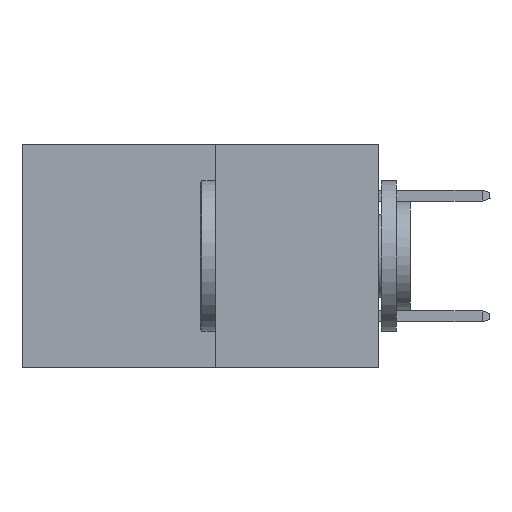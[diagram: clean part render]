
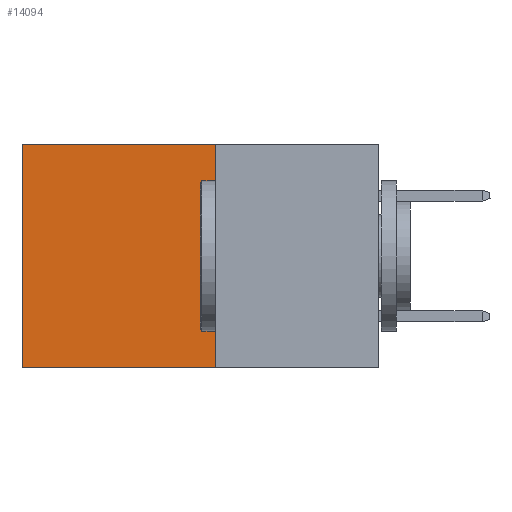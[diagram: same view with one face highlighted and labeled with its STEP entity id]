
A CAD part, left-side view. The second image highlights one B-rep face of the part: STEP entity #14094.
In plain terms, the highlighted planar face has unit normal (-1, 0, 0).
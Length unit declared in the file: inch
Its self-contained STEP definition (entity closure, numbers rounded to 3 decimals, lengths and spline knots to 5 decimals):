
#28 = EDGE_CURVE ( 'NONE', #3592, #15575, #336, .T. ) ;
#336 = LINE ( 'NONE', #8841, #6875 ) ;
#802 = CARTESIAN_POINT ( 'NONE',  ( 0.277, 0.27, -0.37 ) ) ;
#3076 = VERTEX_POINT ( 'NONE', #15320 ) ;
#3592 = VERTEX_POINT ( 'NONE', #4656 ) ;
#4286 = VECTOR ( 'NONE', #13665, 39.37008 ) ;
#4590 = VERTEX_POINT ( 'NONE', #9076 ) ;
#4656 = CARTESIAN_POINT ( 'NONE',  ( 0.277, 0.27, 0. ) ) ;
#4761 = DIRECTION ( 'NONE',  ( 1., 0., 0. ) ) ;
#4862 = EDGE_LOOP ( 'NONE', ( #8521, #10199, #15410, #13033 ) ) ;
#5382 = AXIS2_PLACEMENT_3D ( 'NONE', #802, #4761, #13871 ) ;
#5578 = EDGE_CURVE ( 'NONE', #15575, #3076, #13869, .T. ) ;
#6430 = EDGE_CURVE ( 'NONE', #3592, #4590, #11149, .T. ) ;
#6875 = VECTOR ( 'NONE', #7155, 39.37008 ) ;
#7155 = DIRECTION ( 'NONE',  ( 0., 0., -1. ) ) ;
#8521 = ORIENTED_EDGE ( 'NONE', *, *, #9033, .T. ) ;
#8841 = CARTESIAN_POINT ( 'NONE',  ( 0.277, 0.27, -0.37 ) ) ;
#8924 = CARTESIAN_POINT ( 'NONE',  ( 0.277, 0.59, -0.37 ) ) ;
#9033 = EDGE_CURVE ( 'NONE', #4590, #3076, #12984, .T. ) ;
#9076 = CARTESIAN_POINT ( 'NONE',  ( 0.277, 0.59, 0. ) ) ;
#10199 = ORIENTED_EDGE ( 'NONE', *, *, #5578, .F. ) ;
#10779 = VECTOR ( 'NONE', #13806, 39.37008 ) ;
#11149 = LINE ( 'NONE', #13830, #4286 ) ;
#11525 = CARTESIAN_POINT ( 'NONE',  ( 0.277, 0.27, -0.37 ) ) ;
#12031 = FACE_OUTER_BOUND ( 'NONE', #4862, .T. ) ;
#12542 = PLANE ( 'NONE',  #5382 ) ;
#12849 = DIRECTION ( 'NONE',  ( 0., 0., -1. ) ) ;
#12984 = LINE ( 'NONE', #8924, #16000 ) ;
#13033 = ORIENTED_EDGE ( 'NONE', *, *, #6430, .T. ) ;
#13474 = CARTESIAN_POINT ( 'NONE',  ( 0.277, 0.27, -0.37 ) ) ;
#13665 = DIRECTION ( 'NONE',  ( 0., 1., 0. ) ) ;
#13806 = DIRECTION ( 'NONE',  ( 0., 1., 0. ) ) ;
#13830 = CARTESIAN_POINT ( 'NONE',  ( 0.277, 0.27, 0. ) ) ;
#13869 = LINE ( 'NONE', #13474, #10779 ) ;
#13871 = DIRECTION ( 'NONE',  ( 0., 0., -1. ) ) ;
#14094 = ADVANCED_FACE ( 'NONE', ( #12031 ), #12542, .F. ) ;
#15320 = CARTESIAN_POINT ( 'NONE',  ( 0.277, 0.59, -0.37 ) ) ;
#15410 = ORIENTED_EDGE ( 'NONE', *, *, #28, .F. ) ;
#15575 = VERTEX_POINT ( 'NONE', #11525 ) ;
#16000 = VECTOR ( 'NONE', #12849, 39.37008 ) ;
